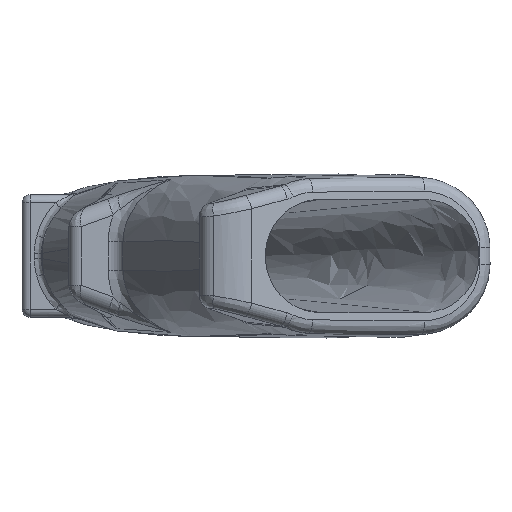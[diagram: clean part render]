
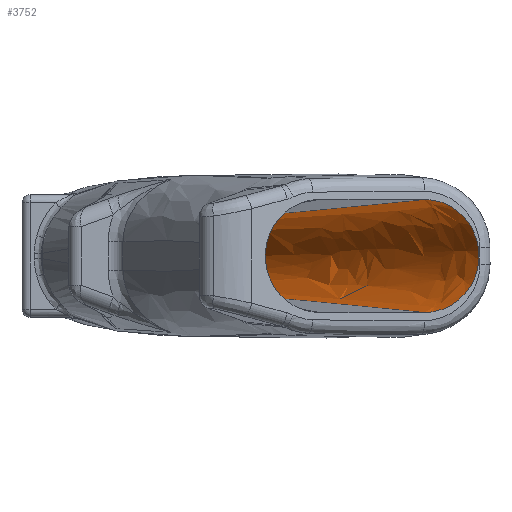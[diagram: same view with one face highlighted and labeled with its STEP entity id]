
A CAD part, front view. The second image highlights one B-rep face of the part: STEP entity #3752.
In plain terms, the highlighted free-form (B-spline) face has degree [3, 1] with [10, 6] control points.
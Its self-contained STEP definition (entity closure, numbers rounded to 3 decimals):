
#40=B_SPLINE_SURFACE_WITH_KNOTS('',3,1,((#8605,#8606,#8607,#8608,#8609,
#8610),(#8611,#8612,#8613,#8614,#8615,#8616),(#8617,#8618,#8619,#8620,#8621,
#8622),(#8623,#8624,#8625,#8626,#8627,#8628),(#8629,#8630,#8631,#8632,#8633,
#8634),(#8635,#8636,#8637,#8638,#8639,#8640),(#8641,#8642,#8643,#8644,#8645,
#8646),(#8647,#8648,#8649,#8650,#8651,#8652),(#8653,#8654,#8655,#8656,#8657,
#8658),(#8659,#8660,#8661,#8662,#8663,#8664)),.UNSPECIFIED.,.F.,.F.,.F.,
(4,2,2,2,4),(2,1,1,1,1,2),(4.971,5.756,6.542,
7.327,8.113),(0.,1.,1.172,1.198,
1.21,1.257),.UNSPECIFIED.);
#661=FACE_OUTER_BOUND('',#885,.T.);
#885=EDGE_LOOP('',(#3135,#3136,#3137,#3138));
#1028=B_SPLINE_CURVE_WITH_KNOTS('',3,(#7171,#7172,#7173,#7174,#7175,#7176,
#7177,#7178,#7179,#7180,#7181,#7182,#7183,#7184,#7185,#7186,#7187,#7188,
#7189,#7190,#7191,#7192),.UNSPECIFIED.,.F.,.F.,(4,2,2,2,2,2,2,2,2,2,4),
(-1.844,-1.74,-1.634,-1.419,
-1.171,-0.922,-0.674,-0.425,
-0.211,-0.105,0.),.UNSPECIFIED.);
#1064=B_SPLINE_CURVE_WITH_KNOTS('',3,(#8667,#8668,#8669,#8670,#8671,#8672,
#8673,#8674,#8675,#8676),.UNSPECIFIED.,.F.,.F.,(4,2,2,2,4),(4.971,
5.756,6.542,7.327,8.113),
 .UNSPECIFIED.);
#1328=LINE('',#8603,#1539);
#1330=LINE('',#8666,#1541);
#1539=VECTOR('',#4691,86.012);
#1541=VECTOR('',#4693,86.012);
#1776=VERTEX_POINT('',#7169);
#1777=VERTEX_POINT('',#7170);
#1834=VERTEX_POINT('',#8602);
#1835=VERTEX_POINT('',#8665);
#2190=EDGE_CURVE('',#1776,#1777,#1028,.T.);
#2304=EDGE_CURVE('',#1834,#1776,#1328,.T.);
#2306=EDGE_CURVE('',#1835,#1777,#1330,.T.);
#2307=EDGE_CURVE('',#1834,#1835,#1064,.T.);
#3135=ORIENTED_EDGE('',*,*,#2190,.T.);
#3136=ORIENTED_EDGE('',*,*,#2306,.F.);
#3137=ORIENTED_EDGE('',*,*,#2307,.F.);
#3138=ORIENTED_EDGE('',*,*,#2304,.T.);
#3752=ADVANCED_FACE('',(#661),#40,.T.);
#4691=DIRECTION('',(-0.537,0.842,-0.052));
#4693=DIRECTION('',(-0.537,0.842,0.052));
#7169=CARTESIAN_POINT('',(28.829,-19.411,6.04));
#7170=CARTESIAN_POINT('',(28.829,-19.411,-6.04));
#7171=CARTESIAN_POINT('Ctrl Pts',(28.829,-19.411,6.04));
#7172=CARTESIAN_POINT('Ctrl Pts',(29.132,-19.236,6.035));
#7173=CARTESIAN_POINT('Ctrl Pts',(29.433,-19.062,5.993));
#7174=CARTESIAN_POINT('Ctrl Pts',(30.027,-18.72,5.838));
#7175=CARTESIAN_POINT('Ctrl Pts',(30.318,-18.552,5.726));
#7176=CARTESIAN_POINT('Ctrl Pts',(31.162,-18.064,5.288));
#7177=CARTESIAN_POINT('Ctrl Pts',(31.672,-17.77,4.868));
#7178=CARTESIAN_POINT('Ctrl Pts',(32.597,-17.235,3.748));
#7179=CARTESIAN_POINT('Ctrl Pts',(32.952,-17.031,3.055));
#7180=CARTESIAN_POINT('Ctrl Pts',(33.441,-16.748,1.583));
#7181=CARTESIAN_POINT('Ctrl Pts',(33.573,-16.672,0.79));
#7182=CARTESIAN_POINT('Ctrl Pts',(33.573,-16.672,-0.79));
#7183=CARTESIAN_POINT('Ctrl Pts',(33.441,-16.748,-1.583));
#7184=CARTESIAN_POINT('Ctrl Pts',(32.952,-17.031,-3.055));
#7185=CARTESIAN_POINT('Ctrl Pts',(32.597,-17.235,-3.748));
#7186=CARTESIAN_POINT('Ctrl Pts',(31.672,-17.77,-4.868));
#7187=CARTESIAN_POINT('Ctrl Pts',(31.162,-18.064,-5.288));
#7188=CARTESIAN_POINT('Ctrl Pts',(30.318,-18.552,-5.726));
#7189=CARTESIAN_POINT('Ctrl Pts',(30.027,-18.72,-5.838));
#7190=CARTESIAN_POINT('Ctrl Pts',(29.433,-19.062,-5.993));
#7191=CARTESIAN_POINT('Ctrl Pts',(29.132,-19.236,-6.035));
#7192=CARTESIAN_POINT('Ctrl Pts',(28.829,-19.411,-6.04));
#8602=CARTESIAN_POINT('',(75.043,-91.813,10.541));
#8603=CARTESIAN_POINT('',(75.043,-91.813,10.541));
#8605=CARTESIAN_POINT('Ctrl Pts',(75.043,-91.813,-10.541));
#8606=CARTESIAN_POINT('Ctrl Pts',(36.782,-31.87,-6.815));
#8607=CARTESIAN_POINT('Ctrl Pts',(30.206,-21.568,-6.174));
#8608=CARTESIAN_POINT('Ctrl Pts',(29.188,-19.972,-6.075));
#8609=CARTESIAN_POINT('Ctrl Pts',(28.729,-19.254,-6.03));
#8610=CARTESIAN_POINT('Ctrl Pts',(26.957,-16.477,-5.858));
#8611=CARTESIAN_POINT('Ctrl Pts',(77.716,-91.097,-10.541));
#8612=CARTESIAN_POINT('Ctrl Pts',(38.584,-31.706,-6.832));
#8613=CARTESIAN_POINT('Ctrl Pts',(31.858,-21.498,-6.194));
#8614=CARTESIAN_POINT('Ctrl Pts',(30.816,-19.917,-6.095));
#8615=CARTESIAN_POINT('Ctrl Pts',(30.347,-19.205,-6.051));
#8616=CARTESIAN_POINT('Ctrl Pts',(28.535,-16.454,-5.879));
#8617=CARTESIAN_POINT('Ctrl Pts',(80.358,-90.389,-9.405));
#8618=CARTESIAN_POINT('Ctrl Pts',(40.403,-31.525,-6.159));
#8619=CARTESIAN_POINT('Ctrl Pts',(33.537,-21.408,-5.602));
#8620=CARTESIAN_POINT('Ctrl Pts',(32.473,-19.841,-5.515));
#8621=CARTESIAN_POINT('Ctrl Pts',(31.994,-19.136,-5.476));
#8622=CARTESIAN_POINT('Ctrl Pts',(30.143,-16.408,-5.326));
#8623=CARTESIAN_POINT('Ctrl Pts',(84.127,-89.379,-5.502));
#8624=CARTESIAN_POINT('Ctrl Pts',(43.066,-31.221,-3.665));
#8625=CARTESIAN_POINT('Ctrl Pts',(36.008,-21.225,-3.35));
#8626=CARTESIAN_POINT('Ctrl Pts',(34.915,-19.677,-3.301));
#8627=CARTESIAN_POINT('Ctrl Pts',(34.423,-18.98,-3.279));
#8628=CARTESIAN_POINT('Ctrl Pts',(32.521,-16.285,-3.194));
#8629=CARTESIAN_POINT('Ctrl Pts',(85.225,-89.085,-2.76));
#8630=CARTESIAN_POINT('Ctrl Pts',(43.873,-31.111,-1.844));
#8631=CARTESIAN_POINT('Ctrl Pts',(36.766,-21.148,-1.687));
#8632=CARTESIAN_POINT('Ctrl Pts',(35.665,-19.604,-1.663));
#8633=CARTESIAN_POINT('Ctrl Pts',(35.169,-18.909,-1.652));
#8634=CARTESIAN_POINT('Ctrl Pts',(33.253,-16.224,-1.609));
#8635=CARTESIAN_POINT('Ctrl Pts',(85.225,-89.085,2.76));
#8636=CARTESIAN_POINT('Ctrl Pts',(43.873,-31.111,1.844));
#8637=CARTESIAN_POINT('Ctrl Pts',(36.766,-21.148,1.687));
#8638=CARTESIAN_POINT('Ctrl Pts',(35.665,-19.604,1.663));
#8639=CARTESIAN_POINT('Ctrl Pts',(35.169,-18.909,1.652));
#8640=CARTESIAN_POINT('Ctrl Pts',(33.253,-16.224,1.609));
#8641=CARTESIAN_POINT('Ctrl Pts',(84.127,-89.379,5.502));
#8642=CARTESIAN_POINT('Ctrl Pts',(43.066,-31.221,3.665));
#8643=CARTESIAN_POINT('Ctrl Pts',(36.008,-21.225,3.35));
#8644=CARTESIAN_POINT('Ctrl Pts',(34.915,-19.677,3.301));
#8645=CARTESIAN_POINT('Ctrl Pts',(34.423,-18.98,3.279));
#8646=CARTESIAN_POINT('Ctrl Pts',(32.521,-16.285,3.194));
#8647=CARTESIAN_POINT('Ctrl Pts',(80.358,-90.389,9.405));
#8648=CARTESIAN_POINT('Ctrl Pts',(40.403,-31.525,6.159));
#8649=CARTESIAN_POINT('Ctrl Pts',(33.537,-21.408,5.602));
#8650=CARTESIAN_POINT('Ctrl Pts',(32.473,-19.841,5.515));
#8651=CARTESIAN_POINT('Ctrl Pts',(31.994,-19.136,5.476));
#8652=CARTESIAN_POINT('Ctrl Pts',(30.143,-16.408,5.326));
#8653=CARTESIAN_POINT('Ctrl Pts',(77.716,-91.097,10.541));
#8654=CARTESIAN_POINT('Ctrl Pts',(38.584,-31.706,6.832));
#8655=CARTESIAN_POINT('Ctrl Pts',(31.858,-21.498,6.194));
#8656=CARTESIAN_POINT('Ctrl Pts',(30.816,-19.917,6.095));
#8657=CARTESIAN_POINT('Ctrl Pts',(30.347,-19.205,6.051));
#8658=CARTESIAN_POINT('Ctrl Pts',(28.535,-16.454,5.879));
#8659=CARTESIAN_POINT('Ctrl Pts',(75.043,-91.813,10.541));
#8660=CARTESIAN_POINT('Ctrl Pts',(36.782,-31.87,6.815));
#8661=CARTESIAN_POINT('Ctrl Pts',(30.206,-21.568,6.174));
#8662=CARTESIAN_POINT('Ctrl Pts',(29.188,-19.972,6.075));
#8663=CARTESIAN_POINT('Ctrl Pts',(28.729,-19.254,6.03));
#8664=CARTESIAN_POINT('Ctrl Pts',(26.957,-16.477,5.858));
#8665=CARTESIAN_POINT('',(75.043,-91.813,-10.541));
#8666=CARTESIAN_POINT('',(75.043,-91.813,-10.541));
#8667=CARTESIAN_POINT('Ctrl Pts',(75.043,-91.813,10.541));
#8668=CARTESIAN_POINT('Ctrl Pts',(77.716,-91.097,10.541));
#8669=CARTESIAN_POINT('Ctrl Pts',(80.358,-90.389,9.405));
#8670=CARTESIAN_POINT('Ctrl Pts',(84.127,-89.379,5.502));
#8671=CARTESIAN_POINT('Ctrl Pts',(85.225,-89.085,2.76));
#8672=CARTESIAN_POINT('Ctrl Pts',(85.225,-89.085,-2.76));
#8673=CARTESIAN_POINT('Ctrl Pts',(84.127,-89.379,-5.502));
#8674=CARTESIAN_POINT('Ctrl Pts',(80.358,-90.389,-9.405));
#8675=CARTESIAN_POINT('Ctrl Pts',(77.716,-91.097,-10.541));
#8676=CARTESIAN_POINT('Ctrl Pts',(75.043,-91.813,-10.541));
